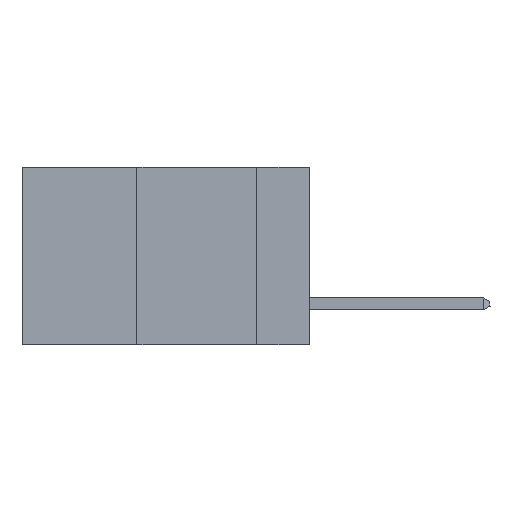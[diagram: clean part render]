
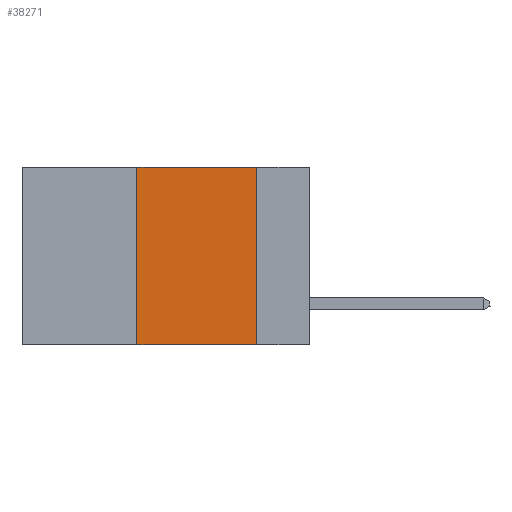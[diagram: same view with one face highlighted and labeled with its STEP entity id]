
A CAD part, left-side view. The second image highlights one B-rep face of the part: STEP entity #38271.
In plain terms, the highlighted planar face has unit normal (-1, 0, 0).
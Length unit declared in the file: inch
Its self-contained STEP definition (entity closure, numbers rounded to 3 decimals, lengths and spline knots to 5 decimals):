
#2288 = CARTESIAN_POINT ( 'NONE',  ( 0., 0.6, -0.37 ) ) ;
#3273 = DIRECTION ( 'NONE',  ( 0., 0., -1. ) ) ;
#3342 = VERTEX_POINT ( 'NONE', #31782 ) ;
#6147 = DIRECTION ( 'NONE',  ( 0., -1., 0. ) ) ;
#6403 = FACE_OUTER_BOUND ( 'NONE', #36532, .T. ) ;
#12095 = DIRECTION ( 'NONE',  ( 0., -1., 0. ) ) ;
#13116 = CARTESIAN_POINT ( 'NONE',  ( 0., 0.11, 0. ) ) ;
#13127 = VECTOR ( 'NONE', #3273, 39.37008 ) ;
#14071 = VECTOR ( 'NONE', #46988, 39.37008 ) ;
#14921 = DIRECTION ( 'NONE',  ( 1., 0., 0. ) ) ;
#16101 = ORIENTED_EDGE ( 'NONE', *, *, #42670, .T. ) ;
#17002 = VERTEX_POINT ( 'NONE', #24337 ) ;
#18107 = ORIENTED_EDGE ( 'NONE', *, *, #44991, .F. ) ;
#19916 = CARTESIAN_POINT ( 'NONE',  ( 0., 0.36, -0.37 ) ) ;
#19968 = LINE ( 'NONE', #46376, #13127 ) ;
#21500 = LINE ( 'NONE', #35844, #14071 ) ;
#22269 = CARTESIAN_POINT ( 'NONE',  ( 0., 0.6, 0. ) ) ;
#24272 = VECTOR ( 'NONE', #12095, 39.37008 ) ;
#24337 = CARTESIAN_POINT ( 'NONE',  ( 0., 0.11, -0.37 ) ) ;
#24504 = ORIENTED_EDGE ( 'NONE', *, *, #35967, .F. ) ;
#25346 = VECTOR ( 'NONE', #6147, 39.37008 ) ;
#25417 = VERTEX_POINT ( 'NONE', #19916 ) ;
#28082 = VERTEX_POINT ( 'NONE', #13116 ) ;
#31782 = CARTESIAN_POINT ( 'NONE',  ( 0., 0.36, 0. ) ) ;
#32838 = AXIS2_PLACEMENT_3D ( 'NONE', #22269, #14921, #33536 ) ;
#33536 = DIRECTION ( 'NONE',  ( 0., 0., -1. ) ) ;
#33903 = LINE ( 'NONE', #45213, #24272 ) ;
#35844 = CARTESIAN_POINT ( 'NONE',  ( 0., 0.36, 0. ) ) ;
#35967 = EDGE_CURVE ( 'NONE', #28082, #17002, #19968, .T. ) ;
#36532 = EDGE_LOOP ( 'NONE', ( #24504, #47183, #18107, #16101 ) ) ;
#38271 = ADVANCED_FACE ( 'NONE', ( #6403 ), #40706, .F. ) ;
#40706 = PLANE ( 'NONE',  #32838 ) ;
#42353 = LINE ( 'NONE', #2288, #25346 ) ;
#42670 = EDGE_CURVE ( 'NONE', #25417, #17002, #42353, .T. ) ;
#44991 = EDGE_CURVE ( 'NONE', #25417, #3342, #21500, .T. ) ;
#45213 = CARTESIAN_POINT ( 'NONE',  ( 0., 0.6, 0. ) ) ;
#45238 = EDGE_CURVE ( 'NONE', #3342, #28082, #33903, .T. ) ;
#46376 = CARTESIAN_POINT ( 'NONE',  ( 0., 0.11, 0. ) ) ;
#46988 = DIRECTION ( 'NONE',  ( 0., 0., 1. ) ) ;
#47183 = ORIENTED_EDGE ( 'NONE', *, *, #45238, .F. ) ;
